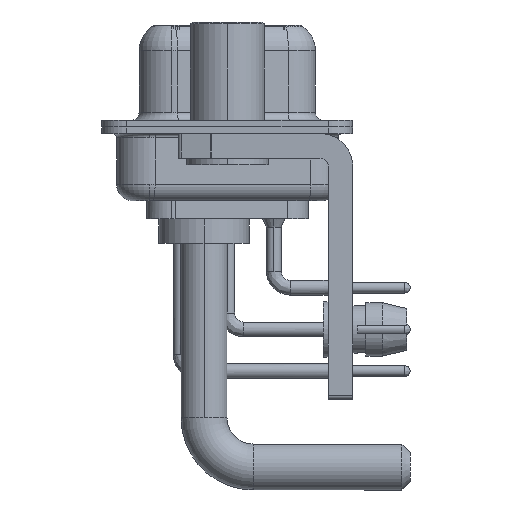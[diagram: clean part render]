
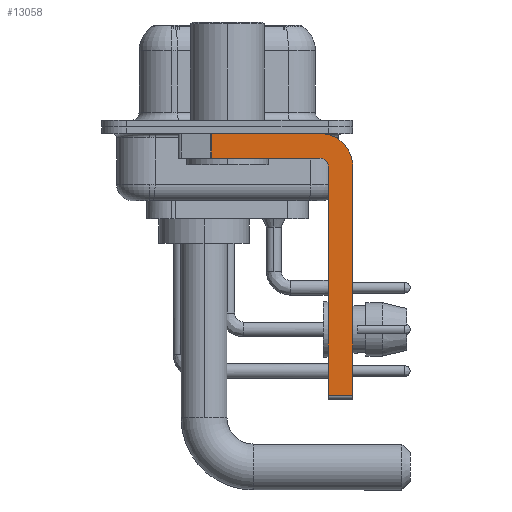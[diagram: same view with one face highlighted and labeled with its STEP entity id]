
A CAD part, left-side view. The second image highlights one B-rep face of the part: STEP entity #13058.
In plain terms, the highlighted planar face has unit normal (-1, 0, 0).
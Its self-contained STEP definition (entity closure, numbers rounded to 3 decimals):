
#657 = PLANE ( 'NONE',  #29649 ) ;
#3379 = CARTESIAN_POINT ( 'NONE',  ( -2.9, -5.65, -1.9 ) ) ;
#3558 = EDGE_CURVE ( 'NONE', #17876, #16267, #28795, .T. ) ;
#3666 = CARTESIAN_POINT ( 'NONE',  ( -2.9, -7.65, -16.35 ) ) ;
#3844 = CARTESIAN_POINT ( 'NONE',  ( -2.9, -7.65, -2.4 ) ) ;
#4975 = EDGE_CURVE ( 'NONE', #32384, #17876, #29238, .T. ) ;
#5427 = DIRECTION ( 'NONE',  ( 0., 0., -1. ) ) ;
#5791 = FACE_OUTER_BOUND ( 'NONE', #22993, .T. ) ;
#5948 = AXIS2_PLACEMENT_3D ( 'NONE', #20081, #14092, #33441 ) ;
#6073 = EDGE_CURVE ( 'NONE', #16937, #16267, #9305, .T. ) ;
#6293 = EDGE_CURVE ( 'NONE', #16937, #24557, #13916, .T. ) ;
#6562 = DIRECTION ( 'NONE',  ( -1., 0., 0. ) ) ;
#8692 = CARTESIAN_POINT ( 'NONE',  ( -2.9, -5.65, -1.9 ) ) ;
#8932 = DIRECTION ( 'NONE',  ( 0., 0., 1. ) ) ;
#9288 = AXIS2_PLACEMENT_3D ( 'NONE', #20399, #6562, #8932 ) ;
#9305 = LINE ( 'NONE', #20407, #10848 ) ;
#10050 = VERTEX_POINT ( 'NONE', #22741 ) ;
#10848 = VECTOR ( 'NONE', #31568, 1000. ) ;
#11041 = CIRCLE ( 'NONE', #9288, 0.5 ) ;
#11195 = CARTESIAN_POINT ( 'NONE',  ( -2.9, -6.15, -16.6 ) ) ;
#13058 = ADVANCED_FACE ( 'NONE', ( #5791 ), #657, .F. ) ;
#13223 = CARTESIAN_POINT ( 'NONE',  ( -2.9, 0.978, -1.9 ) ) ;
#13839 = CARTESIAN_POINT ( 'NONE',  ( -2.9, 3., -0.4 ) ) ;
#13916 = LINE ( 'NONE', #11195, #21322 ) ;
#14092 = DIRECTION ( 'NONE',  ( 1., 0., 0. ) ) ;
#14908 = EDGE_CURVE ( 'NONE', #24557, #25280, #11041, .T. ) ;
#15135 = CARTESIAN_POINT ( 'NONE',  ( -2.9, 0.978, -1.9 ) ) ;
#15917 = ORIENTED_EDGE ( 'NONE', *, *, #3558, .F. ) ;
#16004 = VECTOR ( 'NONE', #22087, 1000. ) ;
#16267 = VERTEX_POINT ( 'NONE', #3666 ) ;
#16937 = VERTEX_POINT ( 'NONE', #21955 ) ;
#17876 = VERTEX_POINT ( 'NONE', #19823 ) ;
#17959 = ORIENTED_EDGE ( 'NONE', *, *, #18323, .F. ) ;
#18051 = LINE ( 'NONE', #15135, #27943 ) ;
#18223 = ORIENTED_EDGE ( 'NONE', *, *, #6073, .T. ) ;
#18323 = EDGE_CURVE ( 'NONE', #25280, #29515, #35883, .T. ) ;
#19823 = CARTESIAN_POINT ( 'NONE',  ( -2.9, -7.65, -2.4 ) ) ;
#19835 = LINE ( 'NONE', #13839, #27060 ) ;
#20081 = CARTESIAN_POINT ( 'NONE',  ( -2.9, -5.65, -2.4 ) ) ;
#20399 = CARTESIAN_POINT ( 'NONE',  ( -2.9, -5.65, -2.4 ) ) ;
#20407 = CARTESIAN_POINT ( 'NONE',  ( -2.9, -5.65, -16.35 ) ) ;
#20950 = EDGE_CURVE ( 'NONE', #10050, #32384, #19835, .T. ) ;
#21294 = ORIENTED_EDGE ( 'NONE', *, *, #14908, .F. ) ;
#21322 = VECTOR ( 'NONE', #22283, 1000. ) ;
#21955 = CARTESIAN_POINT ( 'NONE',  ( -2.9, -6.15, -16.35 ) ) ;
#22087 = DIRECTION ( 'NONE',  ( 0., 0., -1. ) ) ;
#22283 = DIRECTION ( 'NONE',  ( 0., 0., 1. ) ) ;
#22698 = DIRECTION ( 'NONE',  ( 1., 0., 0. ) ) ;
#22741 = CARTESIAN_POINT ( 'NONE',  ( -2.9, 0.978, -0.4 ) ) ;
#22993 = EDGE_LOOP ( 'NONE', ( #26398, #25050, #17959, #21294, #29599, #18223, #15917, #34221 ) ) ;
#24557 = VERTEX_POINT ( 'NONE', #32775 ) ;
#25050 = ORIENTED_EDGE ( 'NONE', *, *, #28438, .T. ) ;
#25280 = VERTEX_POINT ( 'NONE', #3379 ) ;
#26113 = CARTESIAN_POINT ( 'NONE',  ( -2.9, -5.65, -0.4 ) ) ;
#26398 = ORIENTED_EDGE ( 'NONE', *, *, #20950, .F. ) ;
#27060 = VECTOR ( 'NONE', #33004, 1000. ) ;
#27943 = VECTOR ( 'NONE', #29352, 1000. ) ;
#28438 = EDGE_CURVE ( 'NONE', #10050, #29515, #18051, .T. ) ;
#28795 = LINE ( 'NONE', #3844, #16004 ) ;
#29238 = CIRCLE ( 'NONE', #5948, 2. ) ;
#29352 = DIRECTION ( 'NONE',  ( 0., 0., -1. ) ) ;
#29515 = VERTEX_POINT ( 'NONE', #13223 ) ;
#29599 = ORIENTED_EDGE ( 'NONE', *, *, #6293, .F. ) ;
#29649 = AXIS2_PLACEMENT_3D ( 'NONE', #33709, #22698, #5427 ) ;
#30489 = VECTOR ( 'NONE', #35709, 1000. ) ;
#31568 = DIRECTION ( 'NONE',  ( 0., -1., 0. ) ) ;
#32384 = VERTEX_POINT ( 'NONE', #26113 ) ;
#32775 = CARTESIAN_POINT ( 'NONE',  ( -2.9, -6.15, -2.4 ) ) ;
#33004 = DIRECTION ( 'NONE',  ( 0., -1., 0. ) ) ;
#33441 = DIRECTION ( 'NONE',  ( 0., 0., -1. ) ) ;
#33709 = CARTESIAN_POINT ( 'NONE',  ( -2.9, -5.65, -2.4 ) ) ;
#34221 = ORIENTED_EDGE ( 'NONE', *, *, #4975, .F. ) ;
#35709 = DIRECTION ( 'NONE',  ( 0., 1., 0. ) ) ;
#35883 = LINE ( 'NONE', #8692, #30489 ) ;
